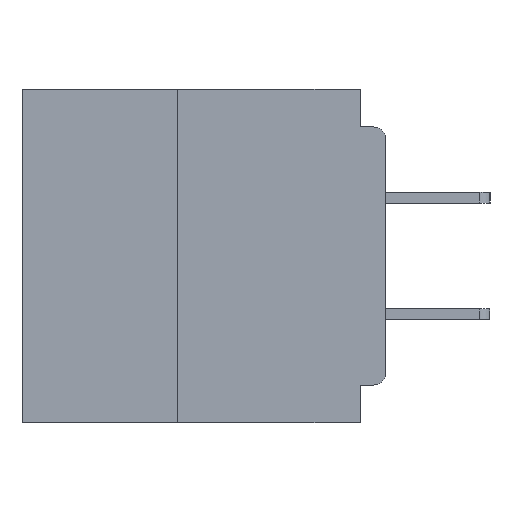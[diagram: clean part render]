
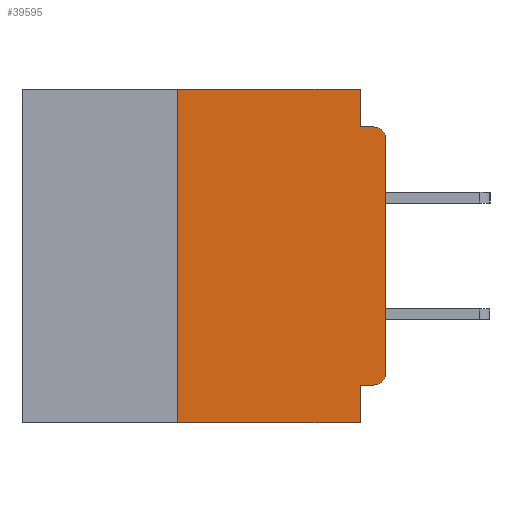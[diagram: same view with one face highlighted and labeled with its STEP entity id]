
A CAD part, left-side view. The second image highlights one B-rep face of the part: STEP entity #39595.
In plain terms, the highlighted planar face has unit normal (-1, 0, 0).
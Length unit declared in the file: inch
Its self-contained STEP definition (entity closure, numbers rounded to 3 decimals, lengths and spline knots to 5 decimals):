
#298 = AXIS2_PLACEMENT_3D ( 'NONE', #5138, #32131, #9072 ) ;
#650 = VERTEX_POINT ( 'NONE', #18356 ) ;
#781 = CARTESIAN_POINT ( 'NONE',  ( 0., 0.031, -0.4 ) ) ;
#2494 = VERTEX_POINT ( 'NONE', #37707 ) ;
#3485 = CIRCLE ( 'NONE', #298, 0.015 ) ;
#3565 = ORIENTED_EDGE ( 'NONE', *, *, #18928, .F. ) ;
#3772 = ORIENTED_EDGE ( 'NONE', *, *, #34280, .F. ) ;
#4054 = VERTEX_POINT ( 'NONE', #6883 ) ;
#4665 = LINE ( 'NONE', #8524, #33050 ) ;
#5013 = ORIENTED_EDGE ( 'NONE', *, *, #32709, .F. ) ;
#5138 = CARTESIAN_POINT ( 'NONE',  ( 0., 0.015, -0.06 ) ) ;
#5652 = CARTESIAN_POINT ( 'NONE',  ( 0., 0.437, 0. ) ) ;
#6601 = CARTESIAN_POINT ( 'NONE',  ( 0., 0., -0.06 ) ) ;
#6883 = CARTESIAN_POINT ( 'NONE',  ( 0., 0.25, 0. ) ) ;
#8524 = CARTESIAN_POINT ( 'NONE',  ( 0., 0., -0.045 ) ) ;
#9072 = DIRECTION ( 'NONE',  ( 0., 0., -1. ) ) ;
#9704 = VERTEX_POINT ( 'NONE', #29943 ) ;
#11306 = CARTESIAN_POINT ( 'NONE',  ( 0., 0.031, -0.4 ) ) ;
#11609 = CARTESIAN_POINT ( 'NONE',  ( 0., 0.25, -0.4 ) ) ;
#11806 = EDGE_CURVE ( 'NONE', #9704, #2494, #4665, .T. ) ;
#11952 = EDGE_CURVE ( 'NONE', #36939, #44609, #27022, .T. ) ;
#12079 = CARTESIAN_POINT ( 'NONE',  ( 0., 0., -0.34 ) ) ;
#12438 = ORIENTED_EDGE ( 'NONE', *, *, #32995, .T. ) ;
#12762 = CARTESIAN_POINT ( 'NONE',  ( 0., 0.015, -0.34 ) ) ;
#13284 = VERTEX_POINT ( 'NONE', #6601 ) ;
#13586 = ORIENTED_EDGE ( 'NONE', *, *, #15447, .F. ) ;
#13745 = FACE_OUTER_BOUND ( 'NONE', #30062, .T. ) ;
#13899 = AXIS2_PLACEMENT_3D ( 'NONE', #5652, #47960, #25067 ) ;
#13957 = DIRECTION ( 'NONE',  ( 0., 0., 1. ) ) ;
#15447 = EDGE_CURVE ( 'NONE', #36939, #4054, #49405, .T. ) ;
#15503 = DIRECTION ( 'NONE',  ( 0., 0., 1. ) ) ;
#16460 = DIRECTION ( 'NONE',  ( 0., -1., 0. ) ) ;
#16641 = DIRECTION ( 'NONE',  ( 0., 0., -1. ) ) ;
#16783 = VECTOR ( 'NONE', #47934, 39.37008 ) ;
#18356 = CARTESIAN_POINT ( 'NONE',  ( 0., 0.031, -0.355 ) ) ;
#18928 = EDGE_CURVE ( 'NONE', #33466, #9704, #32341, .T. ) ;
#19112 = VERTEX_POINT ( 'NONE', #12079 ) ;
#21449 = ORIENTED_EDGE ( 'NONE', *, *, #35828, .T. ) ;
#24268 = ORIENTED_EDGE ( 'NONE', *, *, #29055, .F. ) ;
#25067 = DIRECTION ( 'NONE',  ( 0., 0., -1. ) ) ;
#25921 = LINE ( 'NONE', #11306, #45065 ) ;
#27022 = LINE ( 'NONE', #44119, #16783 ) ;
#28139 = VECTOR ( 'NONE', #35873, 39.37008 ) ;
#28589 = CARTESIAN_POINT ( 'NONE',  ( 0., 0.015, -0.355 ) ) ;
#28975 = ORIENTED_EDGE ( 'NONE', *, *, #11806, .F. ) ;
#29055 = EDGE_CURVE ( 'NONE', #34940, #650, #34072, .T. ) ;
#29092 = VECTOR ( 'NONE', #15503, 39.37008 ) ;
#29943 = CARTESIAN_POINT ( 'NONE',  ( 0., 0.031, -0.045 ) ) ;
#29991 = CARTESIAN_POINT ( 'NONE',  ( 0., 0., -0.355 ) ) ;
#30062 = EDGE_LOOP ( 'NONE', ( #21449, #12438, #28975, #3565, #3772, #13586, #38205, #5013, #24268, #44189 ) ) ;
#30271 = DIRECTION ( 'NONE',  ( 0., 0., -1. ) ) ;
#32131 = DIRECTION ( 'NONE',  ( -1., 0., 0. ) ) ;
#32341 = LINE ( 'NONE', #38054, #42522 ) ;
#32709 = EDGE_CURVE ( 'NONE', #650, #44609, #25921, .T. ) ;
#32995 = EDGE_CURVE ( 'NONE', #13284, #2494, #3485, .T. ) ;
#33042 = AXIS2_PLACEMENT_3D ( 'NONE', #12762, #39693, #16641 ) ;
#33050 = VECTOR ( 'NONE', #16460, 39.37008 ) ;
#33466 = VERTEX_POINT ( 'NONE', #38843 ) ;
#33883 = DIRECTION ( 'NONE',  ( 0., 1., 0. ) ) ;
#34072 = LINE ( 'NONE', #29991, #43004 ) ;
#34280 = EDGE_CURVE ( 'NONE', #4054, #33466, #39579, .T. ) ;
#34379 = DIRECTION ( 'NONE',  ( 0., 0., -1. ) ) ;
#34940 = VERTEX_POINT ( 'NONE', #28589 ) ;
#35828 = EDGE_CURVE ( 'NONE', #19112, #13284, #40012, .T. ) ;
#35873 = DIRECTION ( 'NONE',  ( 0., -1., 0. ) ) ;
#36042 = CARTESIAN_POINT ( 'NONE',  ( 0., 0.437, 0. ) ) ;
#36939 = VERTEX_POINT ( 'NONE', #47351 ) ;
#37707 = CARTESIAN_POINT ( 'NONE',  ( 0., 0.015, -0.045 ) ) ;
#38054 = CARTESIAN_POINT ( 'NONE',  ( 0., 0.031, 0. ) ) ;
#38205 = ORIENTED_EDGE ( 'NONE', *, *, #11952, .T. ) ;
#38843 = CARTESIAN_POINT ( 'NONE',  ( 0., 0.031, 0. ) ) ;
#39579 = LINE ( 'NONE', #36042, #28139 ) ;
#39595 = ADVANCED_FACE ( 'NONE', ( #13745 ), #40374, .F. ) ;
#39693 = DIRECTION ( 'NONE',  ( -1., 0., 0. ) ) ;
#40012 = LINE ( 'NONE', #44635, #48878 ) ;
#40374 = PLANE ( 'NONE',  #13899 ) ;
#42522 = VECTOR ( 'NONE', #30271, 39.37008 ) ;
#43004 = VECTOR ( 'NONE', #33883, 39.37008 ) ;
#43342 = CIRCLE ( 'NONE', #33042, 0.015 ) ;
#44003 = EDGE_CURVE ( 'NONE', #34940, #19112, #43342, .T. ) ;
#44119 = CARTESIAN_POINT ( 'NONE',  ( 0., 0.437, -0.4 ) ) ;
#44189 = ORIENTED_EDGE ( 'NONE', *, *, #44003, .T. ) ;
#44609 = VERTEX_POINT ( 'NONE', #781 ) ;
#44635 = CARTESIAN_POINT ( 'NONE',  ( 0., 0., 0. ) ) ;
#45065 = VECTOR ( 'NONE', #34379, 39.37008 ) ;
#47351 = CARTESIAN_POINT ( 'NONE',  ( 0., 0.25, -0.4 ) ) ;
#47934 = DIRECTION ( 'NONE',  ( 0., -1., 0. ) ) ;
#47960 = DIRECTION ( 'NONE',  ( 1., 0., 0. ) ) ;
#48878 = VECTOR ( 'NONE', #13957, 39.37008 ) ;
#49405 = LINE ( 'NONE', #11609, #29092 ) ;
